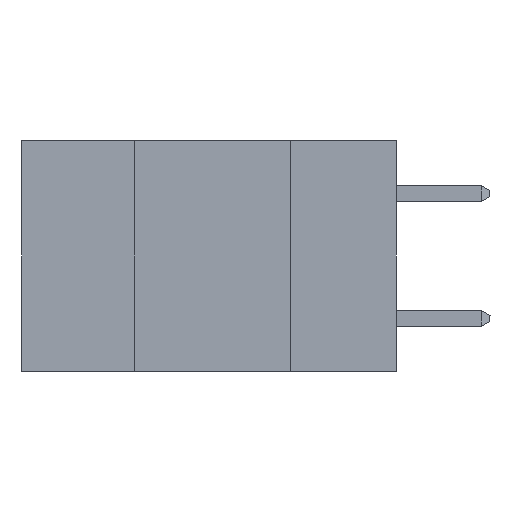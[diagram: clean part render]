
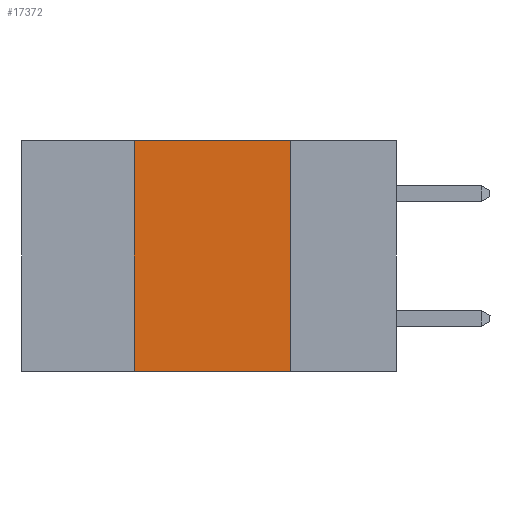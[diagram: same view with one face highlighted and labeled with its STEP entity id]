
A CAD part, left-side view. The second image highlights one B-rep face of the part: STEP entity #17372.
In plain terms, the highlighted planar face has unit normal (-1, 0, 0).
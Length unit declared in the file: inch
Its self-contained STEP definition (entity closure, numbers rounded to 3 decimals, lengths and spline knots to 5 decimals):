
#1166 = EDGE_CURVE ( 'NONE', #12975, #17247, #5754, .T. ) ;
#1796 = CARTESIAN_POINT ( 'NONE',  ( 0., 0.17, -0.37 ) ) ;
#1957 = DIRECTION ( 'NONE',  ( 0., -1., 0. ) ) ;
#2824 = DIRECTION ( 'NONE',  ( 0., -1., 0. ) ) ;
#3614 = ORIENTED_EDGE ( 'NONE', *, *, #16856, .T. ) ;
#3651 = LINE ( 'NONE', #12597, #10274 ) ;
#3881 = VECTOR ( 'NONE', #1957, 39.37008 ) ;
#4415 = CARTESIAN_POINT ( 'NONE',  ( 0., 0.42, 0. ) ) ;
#4543 = EDGE_LOOP ( 'NONE', ( #11734, #15390, #14544, #3614 ) ) ;
#4598 = DIRECTION ( 'NONE',  ( 0., 0., 1. ) ) ;
#4604 = VERTEX_POINT ( 'NONE', #1796 ) ;
#4804 = CARTESIAN_POINT ( 'NONE',  ( 0., 0.6, -0.37 ) ) ;
#5754 = LINE ( 'NONE', #16119, #9486 ) ;
#7512 = CARTESIAN_POINT ( 'NONE',  ( 0., 0.6, 0. ) ) ;
#8254 = CARTESIAN_POINT ( 'NONE',  ( 0., 0.17, 0. ) ) ;
#8868 = PLANE ( 'NONE',  #14108 ) ;
#8924 = DIRECTION ( 'NONE',  ( 0., 0., -1. ) ) ;
#9486 = VECTOR ( 'NONE', #4598, 39.37008 ) ;
#9713 = CARTESIAN_POINT ( 'NONE',  ( 0., 0.42, -0.37 ) ) ;
#9985 = VERTEX_POINT ( 'NONE', #8254 ) ;
#10274 = VECTOR ( 'NONE', #2824, 39.37008 ) ;
#11378 = LINE ( 'NONE', #4804, #3881 ) ;
#11578 = VECTOR ( 'NONE', #14298, 39.37008 ) ;
#11734 = ORIENTED_EDGE ( 'NONE', *, *, #14457, .F. ) ;
#12597 = CARTESIAN_POINT ( 'NONE',  ( 0., 0.6, 0. ) ) ;
#12911 = CARTESIAN_POINT ( 'NONE',  ( 0., 0.17, -0.37 ) ) ;
#12975 = VERTEX_POINT ( 'NONE', #9713 ) ;
#13698 = FACE_OUTER_BOUND ( 'NONE', #4543, .T. ) ;
#14108 = AXIS2_PLACEMENT_3D ( 'NONE', #7512, #17117, #8924 ) ;
#14298 = DIRECTION ( 'NONE',  ( 0., 0., -1. ) ) ;
#14457 = EDGE_CURVE ( 'NONE', #9985, #4604, #15666, .T. ) ;
#14544 = ORIENTED_EDGE ( 'NONE', *, *, #1166, .F. ) ;
#15390 = ORIENTED_EDGE ( 'NONE', *, *, #17161, .F. ) ;
#15666 = LINE ( 'NONE', #12911, #11578 ) ;
#16119 = CARTESIAN_POINT ( 'NONE',  ( 0., 0.42, -0.37 ) ) ;
#16856 = EDGE_CURVE ( 'NONE', #12975, #4604, #11378, .T. ) ;
#17117 = DIRECTION ( 'NONE',  ( 1., 0., 0. ) ) ;
#17161 = EDGE_CURVE ( 'NONE', #17247, #9985, #3651, .T. ) ;
#17247 = VERTEX_POINT ( 'NONE', #4415 ) ;
#17372 = ADVANCED_FACE ( 'NONE', ( #13698 ), #8868, .F. ) ;
